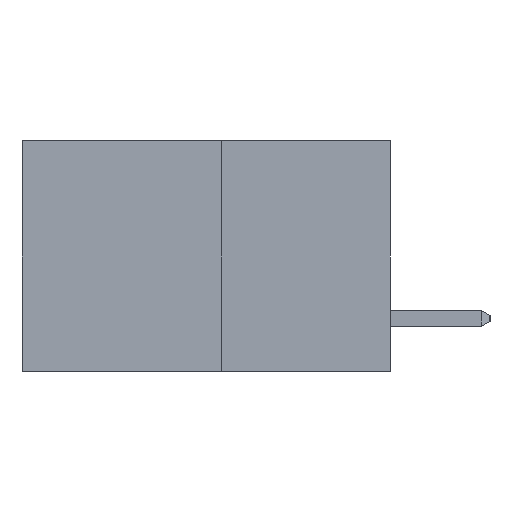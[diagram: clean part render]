
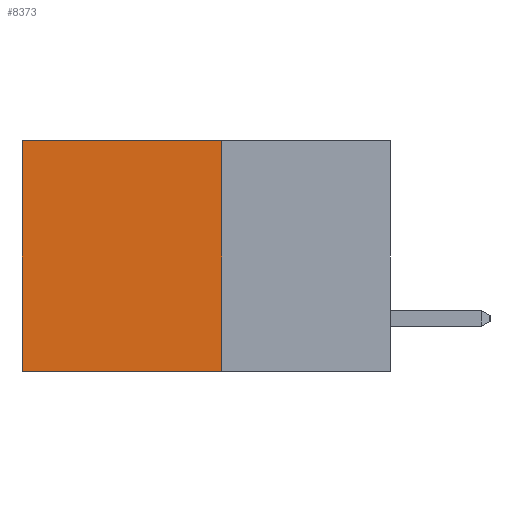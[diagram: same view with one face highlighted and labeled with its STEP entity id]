
A CAD part, left-side view. The second image highlights one B-rep face of the part: STEP entity #8373.
In plain terms, the highlighted planar face has unit normal (-1, 0, 0).
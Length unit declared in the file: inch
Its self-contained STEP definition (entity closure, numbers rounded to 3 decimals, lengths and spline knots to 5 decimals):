
#713 = DIRECTION ( 'NONE',  ( 0., 1., 0. ) ) ;
#797 = CARTESIAN_POINT ( 'NONE',  ( 0.277, 0.27, 0. ) ) ;
#916 = DIRECTION ( 'NONE',  ( 0., 0., -1. ) ) ;
#2031 = LINE ( 'NONE', #13187, #23962 ) ;
#4005 = PLANE ( 'NONE',  #26017 ) ;
#4871 = DIRECTION ( 'NONE',  ( 0., 1., 0. ) ) ;
#5101 = CARTESIAN_POINT ( 'NONE',  ( 0.277, 0.27, 0. ) ) ;
#6180 = LINE ( 'NONE', #797, #16510 ) ;
#6342 = ORIENTED_EDGE ( 'NONE', *, *, #8323, .F. ) ;
#6893 = VERTEX_POINT ( 'NONE', #7335 ) ;
#7335 = CARTESIAN_POINT ( 'NONE',  ( 0.277, 0.27, -0.37 ) ) ;
#7771 = VECTOR ( 'NONE', #713, 39.37008 ) ;
#7969 = FACE_OUTER_BOUND ( 'NONE', #23603, .T. ) ;
#8167 = CARTESIAN_POINT ( 'NONE',  ( 0.277, 0.27, -0.37 ) ) ;
#8323 = EDGE_CURVE ( 'NONE', #12432, #6893, #24438, .T. ) ;
#8373 = ADVANCED_FACE ( 'NONE', ( #7969 ), #4005, .F. ) ;
#9215 = VERTEX_POINT ( 'NONE', #21418 ) ;
#10205 = DIRECTION ( 'NONE',  ( 0., 0., -1. ) ) ;
#11099 = EDGE_CURVE ( 'NONE', #18532, #9215, #2031, .T. ) ;
#11732 = EDGE_CURVE ( 'NONE', #6893, #9215, #18751, .T. ) ;
#12077 = ORIENTED_EDGE ( 'NONE', *, *, #11732, .F. ) ;
#12112 = CARTESIAN_POINT ( 'NONE',  ( 0.277, 0.27, -0.37 ) ) ;
#12432 = VERTEX_POINT ( 'NONE', #5101 ) ;
#13187 = CARTESIAN_POINT ( 'NONE',  ( 0.277, 0.59, -0.37 ) ) ;
#14203 = DIRECTION ( 'NONE',  ( 0., 0., -1. ) ) ;
#16510 = VECTOR ( 'NONE', #4871, 39.37008 ) ;
#16949 = CARTESIAN_POINT ( 'NONE',  ( 0.277, 0.59, 0. ) ) ;
#18078 = ORIENTED_EDGE ( 'NONE', *, *, #19896, .T. ) ;
#18532 = VERTEX_POINT ( 'NONE', #16949 ) ;
#18751 = LINE ( 'NONE', #23301, #7771 ) ;
#19582 = VECTOR ( 'NONE', #14203, 39.37008 ) ;
#19896 = EDGE_CURVE ( 'NONE', #12432, #18532, #6180, .T. ) ;
#21418 = CARTESIAN_POINT ( 'NONE',  ( 0.277, 0.59, -0.37 ) ) ;
#21905 = ORIENTED_EDGE ( 'NONE', *, *, #11099, .T. ) ;
#22614 = DIRECTION ( 'NONE',  ( 1., 0., 0. ) ) ;
#23301 = CARTESIAN_POINT ( 'NONE',  ( 0.277, 0.27, -0.37 ) ) ;
#23603 = EDGE_LOOP ( 'NONE', ( #21905, #12077, #6342, #18078 ) ) ;
#23962 = VECTOR ( 'NONE', #916, 39.37008 ) ;
#24438 = LINE ( 'NONE', #12112, #19582 ) ;
#26017 = AXIS2_PLACEMENT_3D ( 'NONE', #8167, #22614, #10205 ) ;
